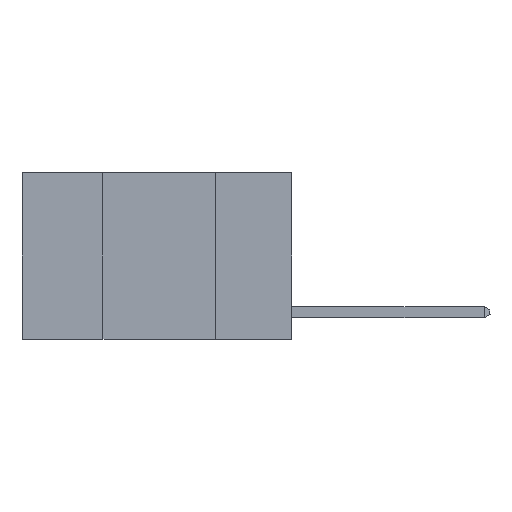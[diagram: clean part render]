
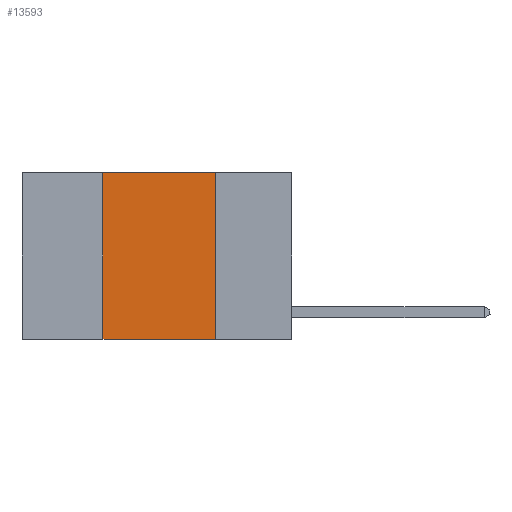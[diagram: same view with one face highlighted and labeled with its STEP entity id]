
A CAD part, left-side view. The second image highlights one B-rep face of the part: STEP entity #13593.
In plain terms, the highlighted planar face has unit normal (-1, 0, 0).
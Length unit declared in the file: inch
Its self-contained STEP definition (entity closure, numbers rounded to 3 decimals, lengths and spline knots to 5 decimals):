
#62 = AXIS2_PLACEMENT_3D ( 'NONE', #78, #13847, #12517 ) ;
#78 = CARTESIAN_POINT ( 'NONE',  ( 0., 0.6, 0. ) ) ;
#385 = EDGE_LOOP ( 'NONE', ( #17369, #15896, #5340, #21215 ) ) ;
#550 = VERTEX_POINT ( 'NONE', #16540 ) ;
#1231 = LINE ( 'NONE', #6502, #16443 ) ;
#4423 = LINE ( 'NONE', #15110, #10772 ) ;
#4605 = VERTEX_POINT ( 'NONE', #20460 ) ;
#4644 = DIRECTION ( 'NONE',  ( 0., -1., 0. ) ) ;
#4807 = CARTESIAN_POINT ( 'NONE',  ( 0., 0.17, 0. ) ) ;
#4976 = DIRECTION ( 'NONE',  ( 0., -1., 0. ) ) ;
#5340 = ORIENTED_EDGE ( 'NONE', *, *, #9601, .F. ) ;
#6502 = CARTESIAN_POINT ( 'NONE',  ( 0., 0.6, 0. ) ) ;
#9246 = CARTESIAN_POINT ( 'NONE',  ( 0., 0.17, 0. ) ) ;
#9601 = EDGE_CURVE ( 'NONE', #550, #4605, #14020, .T. ) ;
#10133 = VERTEX_POINT ( 'NONE', #9246 ) ;
#10772 = VECTOR ( 'NONE', #4644, 39.37008 ) ;
#12105 = DIRECTION ( 'NONE',  ( 0., 0., -1. ) ) ;
#12411 = PLANE ( 'NONE',  #62 ) ;
#12517 = DIRECTION ( 'NONE',  ( 0., 0., -1. ) ) ;
#12815 = VECTOR ( 'NONE', #12105, 39.37008 ) ;
#12997 = EDGE_CURVE ( 'NONE', #10133, #14829, #15500, .T. ) ;
#13422 = VECTOR ( 'NONE', #21248, 39.37008 ) ;
#13593 = ADVANCED_FACE ( 'NONE', ( #17366 ), #12411, .F. ) ;
#13847 = DIRECTION ( 'NONE',  ( 1., 0., 0. ) ) ;
#14020 = LINE ( 'NONE', #19139, #13422 ) ;
#14829 = VERTEX_POINT ( 'NONE', #23039 ) ;
#15110 = CARTESIAN_POINT ( 'NONE',  ( 0., 0.6, -0.37 ) ) ;
#15500 = LINE ( 'NONE', #4807, #12815 ) ;
#15896 = ORIENTED_EDGE ( 'NONE', *, *, #22499, .F. ) ;
#16443 = VECTOR ( 'NONE', #4976, 39.37008 ) ;
#16540 = CARTESIAN_POINT ( 'NONE',  ( 0., 0.42, -0.37 ) ) ;
#17366 = FACE_OUTER_BOUND ( 'NONE', #385, .T. ) ;
#17369 = ORIENTED_EDGE ( 'NONE', *, *, #12997, .F. ) ;
#19139 = CARTESIAN_POINT ( 'NONE',  ( 0., 0.42, 0. ) ) ;
#20460 = CARTESIAN_POINT ( 'NONE',  ( 0., 0.42, 0. ) ) ;
#21215 = ORIENTED_EDGE ( 'NONE', *, *, #21926, .T. ) ;
#21248 = DIRECTION ( 'NONE',  ( 0., 0., 1. ) ) ;
#21926 = EDGE_CURVE ( 'NONE', #550, #14829, #4423, .T. ) ;
#22499 = EDGE_CURVE ( 'NONE', #4605, #10133, #1231, .T. ) ;
#23039 = CARTESIAN_POINT ( 'NONE',  ( 0., 0.17, -0.37 ) ) ;
